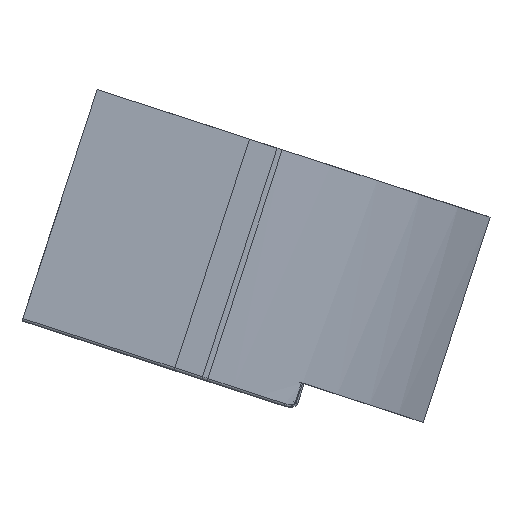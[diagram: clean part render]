
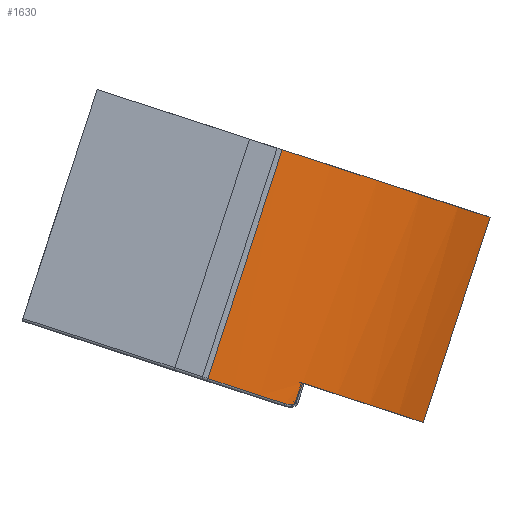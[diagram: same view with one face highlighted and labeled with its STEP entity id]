
A CAD part, front view. The second image highlights one B-rep face of the part: STEP entity #1630.
In plain terms, the highlighted cylindrical face has radius 10.895 mm (diameter 21.791 mm), a partial arc.
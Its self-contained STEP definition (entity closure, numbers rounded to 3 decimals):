
#100=FACE_OUTER_BOUND('',#186,.T.);
#186=EDGE_LOOP('',(#1244,#1245,#1246,#1247,#1248,#1249,#1250));
#254=B_SPLINE_CURVE_WITH_KNOTS('',3,(#2673,#2674,#2675,#2676,#2677,#2678,
#2679,#2680,#2681,#2682,#2683),.UNSPECIFIED.,.F.,.F.,(4,1,1,1,1,1,1,1,4),
(0.,0.002,0.003,0.007,
0.01,0.013,0.02,0.033,
0.046),.UNSPECIFIED.);
#272=CIRCLE('',#1723,10.895);
#285=CIRCLE('',#1745,10.895);
#289=CIRCLE('',#1753,10.895);
#382=LINE('',#2537,#572);
#386=LINE('',#2701,#576);
#387=LINE('',#2705,#577);
#572=VECTOR('',#2000,10.);
#576=VECTOR('',#2024,10.);
#577=VECTOR('',#2029,10.);
#739=VERTEX_POINT('',#2443);
#740=VERTEX_POINT('',#2445);
#778=VERTEX_POINT('',#2533);
#780=VERTEX_POINT('',#2615);
#782=VERTEX_POINT('',#2685);
#786=VERTEX_POINT('',#2700);
#787=VERTEX_POINT('',#2704);
#909=EDGE_CURVE('',#739,#740,#272,.T.);
#954=EDGE_CURVE('',#740,#778,#382,.T.);
#957=EDGE_CURVE('',#778,#780,#254,.T.);
#960=EDGE_CURVE('',#780,#782,#285,.T.);
#966=EDGE_CURVE('',#786,#782,#386,.T.);
#968=EDGE_CURVE('',#787,#739,#387,.T.);
#969=EDGE_CURVE('',#787,#786,#289,.T.);
#1244=ORIENTED_EDGE('',*,*,#960,.F.);
#1245=ORIENTED_EDGE('',*,*,#957,.F.);
#1246=ORIENTED_EDGE('',*,*,#954,.F.);
#1247=ORIENTED_EDGE('',*,*,#909,.F.);
#1248=ORIENTED_EDGE('',*,*,#968,.F.);
#1249=ORIENTED_EDGE('',*,*,#969,.T.);
#1250=ORIENTED_EDGE('',*,*,#966,.T.);
#1593=CYLINDRICAL_SURFACE('',#1752,10.895);
#1630=ADVANCED_FACE('',(#100),#1593,.T.);
#1723=AXIS2_PLACEMENT_3D('',#2446,#1930,#1931);
#1745=AXIS2_PLACEMENT_3D('',#2689,#2009,#2010);
#1752=AXIS2_PLACEMENT_3D('',#2703,#2027,#2028);
#1753=AXIS2_PLACEMENT_3D('',#2706,#2030,#2031);
#1930=DIRECTION('center_axis',(-0.309,0.,
-0.951));
#1931=DIRECTION('ref_axis',(0.773,-0.583,-0.251));
#2000=DIRECTION('',(-0.309,0.,-0.951));
#2009=DIRECTION('center_axis',(-0.309,0.,
-0.951));
#2010=DIRECTION('ref_axis',(0.224,-0.972,-0.073));
#2024=DIRECTION('',(-0.309,0.,-0.951));
#2027=DIRECTION('center_axis',(-0.309,0.,
-0.951));
#2028=DIRECTION('ref_axis',(0.773,-0.583,-0.251));
#2029=DIRECTION('',(-0.309,0.,-0.951));
#2030=DIRECTION('center_axis',(-0.309,0.,
-0.951));
#2031=DIRECTION('ref_axis',(0.773,-0.583,-0.251));
#2443=CARTESIAN_POINT('',(-13.439,15.574,63.245));
#2445=CARTESIAN_POINT('',(-17.808,11.899,64.664));
#2446=CARTESIAN_POINT('Origin',(-21.857,21.928,65.98));
#2533=CARTESIAN_POINT('',(-18.039,11.899,63.951));
#2537=CARTESIAN_POINT('',(-15.397,11.899,72.083));
#2615=CARTESIAN_POINT('',(-18.443,11.748,63.924));
#2673=CARTESIAN_POINT('Ctrl Pts',(-18.039,11.899,63.951));
#2674=CARTESIAN_POINT('Ctrl Pts',(-18.041,11.899,63.946));
#2675=CARTESIAN_POINT('Ctrl Pts',(-18.046,11.898,63.936));
#2676=CARTESIAN_POINT('Ctrl Pts',(-18.06,11.895,63.919));
#2677=CARTESIAN_POINT('Ctrl Pts',(-18.082,11.888,63.904));
#2678=CARTESIAN_POINT('Ctrl Pts',(-18.111,11.878,63.893));
#2679=CARTESIAN_POINT('Ctrl Pts',(-18.152,11.863,63.884));
#2680=CARTESIAN_POINT('Ctrl Pts',(-18.223,11.835,63.879));
#2681=CARTESIAN_POINT('Ctrl Pts',(-18.325,11.795,63.891));
#2682=CARTESIAN_POINT('Ctrl Pts',(-18.404,11.763,63.912));
#2683=CARTESIAN_POINT('Ctrl Pts',(-18.443,11.748,63.924));
#2685=CARTESIAN_POINT('',(-21.231,11.074,64.83));
#2689=CARTESIAN_POINT('Origin',(-22.135,21.928,65.124));
#2700=CARTESIAN_POINT('',(-18.542,11.074,73.104));
#2701=CARTESIAN_POINT('',(-18.542,11.074,73.104));
#2703=CARTESIAN_POINT('Origin',(-19.447,21.928,73.398));
#2704=CARTESIAN_POINT('',(-11.029,15.574,70.663));
#2705=CARTESIAN_POINT('',(-11.029,15.574,70.663));
#2706=CARTESIAN_POINT('Origin',(-19.447,21.928,73.398));
